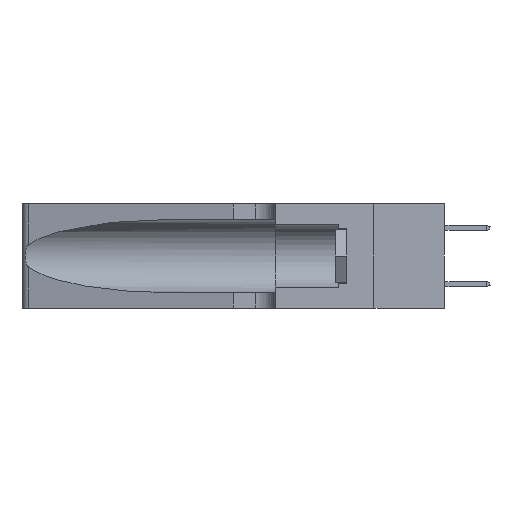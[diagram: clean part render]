
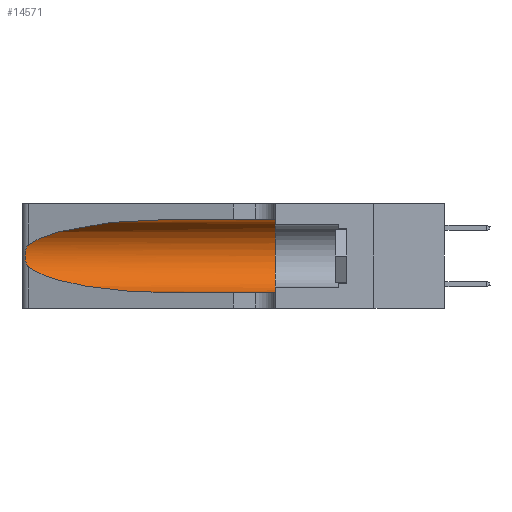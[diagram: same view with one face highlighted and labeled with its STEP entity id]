
A CAD part, left-side view. The second image highlights one B-rep face of the part: STEP entity #14571.
In plain terms, the highlighted cylindrical face has radius 3.308 mm (diameter 6.617 mm), a partial arc.
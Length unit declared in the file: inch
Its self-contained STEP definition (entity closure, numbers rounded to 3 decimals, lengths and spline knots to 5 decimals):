
#142 = DIRECTION ( 'NONE',  ( 0., 1., 0. ) ) ;
#248 = CARTESIAN_POINT ( 'NONE',  ( 0.1305, 1.61858, 0.185 ) ) ;
#311 = CARTESIAN_POINT ( 'NONE',  ( 0.25487, 1.22718, 0.14631 ) ) ;
#1376 = VERTEX_POINT ( 'NONE', #21586 ) ;
#2037 = FACE_OUTER_BOUND ( 'NONE', #7434, .T. ) ;
#2246 = ORIENTED_EDGE ( 'NONE', *, *, #27823, .F. ) ;
#3089 = CARTESIAN_POINT ( 'NONE',  ( 0.25639, 1.23184, 0.21858 ) ) ;
#3116 = CIRCLE ( 'NONE', #25114, 0.13025 ) ;
#3758 = CARTESIAN_POINT ( 'NONE',  ( 0.2373, 1.15595, 0.08982 ) ) ;
#5153 = VERTEX_POINT ( 'NONE', #13891 ) ;
#5965 = CARTESIAN_POINT ( 'NONE',  ( 0.25854, 1.2359, 0.20912 ) ) ;
#6412 = CARTESIAN_POINT ( 'NONE',  ( 0.18966, 0.96281, 0.31525 ) ) ;
#6556 = VECTOR ( 'NONE', #20570, 39.37008 ) ;
#6650 = CARTESIAN_POINT ( 'NONE',  ( 0.25487, 1.22718, 0.14631 ) ) ;
#7434 = EDGE_LOOP ( 'NONE', ( #35874, #20058, #28329, #17965, #2246, #15393 ) ) ;
#8876 = CARTESIAN_POINT ( 'NONE',  ( 0.26075, 1.23896, 0.19203 ) ) ;
#10782 = DIRECTION ( 'NONE',  ( 0., -1., 0. ) ) ;
#10904 = VERTEX_POINT ( 'NONE', #21546 ) ;
#11713 = CARTESIAN_POINT ( 'NONE',  ( 0.26017, 1.23833, 0.17102 ) ) ;
#12018 = CARTESIAN_POINT ( 'NONE',  ( 0.1305, 0.72297, 0.31525 ) ) ;
#12138 = CARTESIAN_POINT ( 'NONE',  ( 0.25487, 1.22718, 0.22369 ) ) ;
#12380 = CARTESIAN_POINT ( 'NONE',  ( 0.18966, 0.96281, 0.05475 ) ) ;
#13409 = EDGE_CURVE ( 'NONE', #1376, #10904, #24511, .T. ) ;
#13891 = CARTESIAN_POINT ( 'NONE',  ( 0.1305, 0.35, 0.05475 ) ) ;
#14090 = LINE ( 'NONE', #26103, #6556 ) ;
#14510 = CARTESIAN_POINT ( 'NONE',  ( 0.25789, 1.23486, 0.15765 ) ) ;
#14571 = ADVANCED_FACE ( 'NONE', ( #2037 ), #23691, .F. ) ;
#15393 = ORIENTED_EDGE ( 'NONE', *, *, #23217, .F. ) ;
#17160 = CARTESIAN_POINT ( 'NONE',  ( 0.1305, 0.35, 0.185 ) ) ;
#17327 = CARTESIAN_POINT ( 'NONE',  ( 0.25555, 1.22993, 0.14849 ) ) ;
#17965 = ORIENTED_EDGE ( 'NONE', *, *, #31714, .T. ) ;
#19081 = CARTESIAN_POINT ( 'NONE',  ( 0.1305, 1.61858, 0.05475 ) ) ;
#19965 = DIRECTION ( 'NONE',  ( 0., 0., 1. ) ) ;
#20058 = ORIENTED_EDGE ( 'NONE', *, *, #13409, .T. ) ;
#20067 = DIRECTION ( 'NONE',  ( 0., 0., -1. ) ) ;
#20570 = DIRECTION ( 'NONE',  ( 0., -1., 0. ) ) ;
#20836 = CARTESIAN_POINT ( 'NONE',  ( 0.1305, 0.72297, 0.31525 ) ) ;
#21013 = VERTEX_POINT ( 'NONE', #20836 ) ;
#21546 = CARTESIAN_POINT ( 'NONE',  ( 0.25487, 1.22718, 0.14631 ) ) ;
#21586 = CARTESIAN_POINT ( 'NONE',  ( 0.25487, 1.22718, 0.22369 ) ) ;
#22725 = CARTESIAN_POINT ( 'NONE',  ( 0.25487, 1.22718, 0.22369 ) ) ;
#22775 = DIRECTION ( 'NONE',  ( 0., -1., 0. ) ) ;
#22842 = CARTESIAN_POINT ( 'NONE',  ( 0.25787, 1.23484, 0.2124 ) ) ;
#22867 = CARTESIAN_POINT ( 'NONE',  ( 0.1305, 0.35, 0.31525 ) ) ;
#23217 = EDGE_CURVE ( 'NONE', #21013, #31924, #14090, .T. ) ;
#23691 = CYLINDRICAL_SURFACE ( 'NONE', #35066, 0.13025 ) ;
#24511 = B_SPLINE_CURVE_WITH_KNOTS ( 'NONE', 3,
 ( #22725, #34003, #3089, #22842, #5965, #25648, #8876, #28484, #11713, #31314, #14510, #34121, #17327, #311 ),
 .UNSPECIFIED., .F., .F.,
 ( 4, 2, 2, 2, 2, 2, 4 ),
 ( 0., 0.00027, 0.00053, 0.00107, 0.0016, 0.00187, 0.00214 ),
 .UNSPECIFIED. ) ;
#25114 = AXIS2_PLACEMENT_3D ( 'NONE', #17160, #142, #19965 ) ;
#25264 = EDGE_CURVE ( 'NONE', #10904, #25573, #34837, .T. ) ;
#25334 = CARTESIAN_POINT ( 'NONE',  ( 0.1305, 0.72297, 0.05475 ) ) ;
#25573 = VERTEX_POINT ( 'NONE', #25334 ) ;
#25648 = CARTESIAN_POINT ( 'NONE',  ( 0.26018, 1.23835, 0.19895 ) ) ;
#26103 = CARTESIAN_POINT ( 'NONE',  ( 0.1305, 1.61858, 0.31525 ) ) ;
#27823 = EDGE_CURVE ( 'NONE', #31924, #5153, #3116, .T. ) ;
#28319 =( BOUNDED_CURVE ( )  B_SPLINE_CURVE ( 3, ( #12018, #6412, #28917, #12138 ),
 .UNSPECIFIED., .F., .F. ) 
 B_SPLINE_CURVE_WITH_KNOTS ( ( 4, 4 ),
 ( 1.5708, 2.84003 ),
 .UNSPECIFIED. ) 
 CURVE ( )  GEOMETRIC_REPRESENTATION_ITEM ( )  RATIONAL_B_SPLINE_CURVE ( ( 1., 0.87, 0.87, 1. ) ) 
 REPRESENTATION_ITEM ( '' )  );
#28329 = ORIENTED_EDGE ( 'NONE', *, *, #25264, .T. ) ;
#28484 = CARTESIAN_POINT ( 'NONE',  ( 0.26075, 1.23896, 0.178 ) ) ;
#28917 = CARTESIAN_POINT ( 'NONE',  ( 0.2373, 1.15595, 0.28018 ) ) ;
#29256 = LINE ( 'NONE', #19081, #35804 ) ;
#31314 = CARTESIAN_POINT ( 'NONE',  ( 0.25856, 1.23593, 0.16098 ) ) ;
#31350 = EDGE_CURVE ( 'NONE', #21013, #1376, #28319, .T. ) ;
#31714 = EDGE_CURVE ( 'NONE', #25573, #5153, #29256, .T. ) ;
#31924 = VERTEX_POINT ( 'NONE', #22867 ) ;
#31974 = CARTESIAN_POINT ( 'NONE',  ( 0.1305, 0.72297, 0.05475 ) ) ;
#34003 = CARTESIAN_POINT ( 'NONE',  ( 0.25555, 1.22994, 0.2215 ) ) ;
#34121 = CARTESIAN_POINT ( 'NONE',  ( 0.25639, 1.23186, 0.15144 ) ) ;
#34837 =( BOUNDED_CURVE ( )  B_SPLINE_CURVE ( 3, ( #6650, #3758, #12380, #31974 ),
 .UNSPECIFIED., .F., .T. ) 
 B_SPLINE_CURVE_WITH_KNOTS ( ( 4, 4 ),
 ( 3.44316, 4.71239 ),
 .UNSPECIFIED. ) 
 CURVE ( )  GEOMETRIC_REPRESENTATION_ITEM ( )  RATIONAL_B_SPLINE_CURVE ( ( 1., 0.87, 0.87, 1. ) ) 
 REPRESENTATION_ITEM ( '' )  );
#35066 = AXIS2_PLACEMENT_3D ( 'NONE', #248, #22775, #20067 ) ;
#35804 = VECTOR ( 'NONE', #10782, 39.37008 ) ;
#35874 = ORIENTED_EDGE ( 'NONE', *, *, #31350, .T. ) ;
